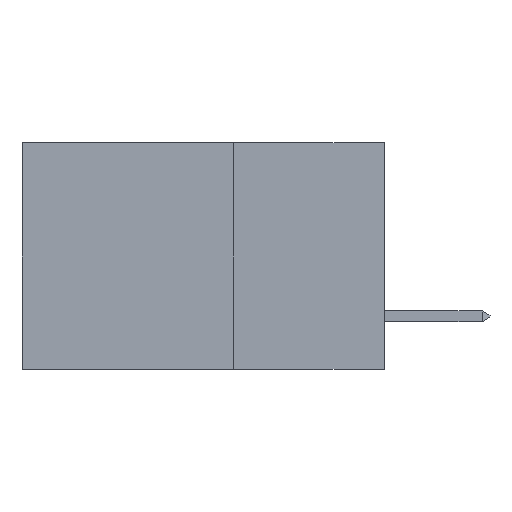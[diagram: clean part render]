
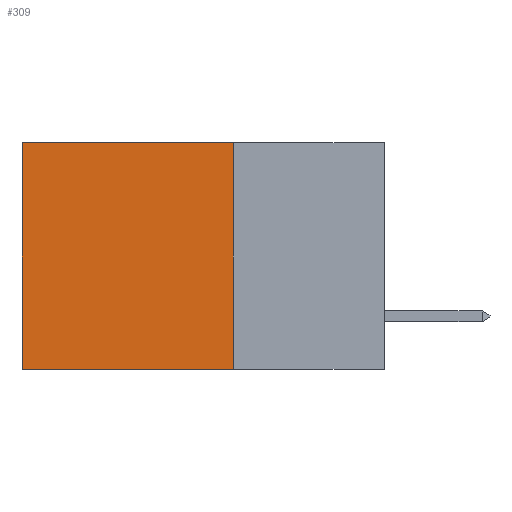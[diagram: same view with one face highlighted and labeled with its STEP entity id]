
A CAD part, left-side view. The second image highlights one B-rep face of the part: STEP entity #309.
In plain terms, the highlighted planar face has unit normal (-1, 0, 0).
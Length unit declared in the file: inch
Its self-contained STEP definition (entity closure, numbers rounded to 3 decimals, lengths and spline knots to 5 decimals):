
#145 = EDGE_CURVE ( 'NONE', #9549, #3495, #621, .T. ) ;
#281 = ORIENTED_EDGE ( 'NONE', *, *, #145, .T. ) ;
#309 = ADVANCED_FACE ( 'NONE', ( #3545 ), #6428, .F. ) ;
#405 = DIRECTION ( 'NONE',  ( 1., 0., 0. ) ) ;
#621 = LINE ( 'NONE', #3149, #6373 ) ;
#1084 = DIRECTION ( 'NONE',  ( 0., 0., -1. ) ) ;
#1146 = ORIENTED_EDGE ( 'NONE', *, *, #4583, .T. ) ;
#1243 = VECTOR ( 'NONE', #5095, 39.37008 ) ;
#1458 = LINE ( 'NONE', #4060, #7192 ) ;
#1569 = LINE ( 'NONE', #3589, #6022 ) ;
#2147 = ORIENTED_EDGE ( 'NONE', *, *, #7926, .F. ) ;
#2743 = DIRECTION ( 'NONE',  ( 0., 0., -1. ) ) ;
#2955 = DIRECTION ( 'NONE',  ( 0., 0., -1. ) ) ;
#3149 = CARTESIAN_POINT ( 'NONE',  ( 0.2875, 0.6, -0.375 ) ) ;
#3495 = VERTEX_POINT ( 'NONE', #4657 ) ;
#3545 = FACE_OUTER_BOUND ( 'NONE', #7083, .T. ) ;
#3589 = CARTESIAN_POINT ( 'NONE',  ( 0.2875, 0.25, -0.375 ) ) ;
#4060 = CARTESIAN_POINT ( 'NONE',  ( 0.2875, 0.25, -0.375 ) ) ;
#4084 = CARTESIAN_POINT ( 'NONE',  ( 0.2875, 0.6, 0. ) ) ;
#4092 = CARTESIAN_POINT ( 'NONE',  ( 0.2875, 0.25, 0. ) ) ;
#4281 = VERTEX_POINT ( 'NONE', #8550 ) ;
#4338 = CARTESIAN_POINT ( 'NONE',  ( 0.2875, 0.25, 0. ) ) ;
#4583 = EDGE_CURVE ( 'NONE', #8973, #9549, #5475, .T. ) ;
#4657 = CARTESIAN_POINT ( 'NONE',  ( 0.2875, 0.6, -0.375 ) ) ;
#4826 = DIRECTION ( 'NONE',  ( 0., 1., 0. ) ) ;
#4952 = CARTESIAN_POINT ( 'NONE',  ( 0.2875, 0.25, -0.375 ) ) ;
#5095 = DIRECTION ( 'NONE',  ( 0., 1., 0. ) ) ;
#5475 = LINE ( 'NONE', #4338, #1243 ) ;
#5564 = AXIS2_PLACEMENT_3D ( 'NONE', #4952, #405, #2743 ) ;
#6022 = VECTOR ( 'NONE', #2955, 39.37008 ) ;
#6373 = VECTOR ( 'NONE', #1084, 39.37008 ) ;
#6428 = PLANE ( 'NONE',  #5564 ) ;
#6469 = EDGE_CURVE ( 'NONE', #8973, #4281, #1569, .T. ) ;
#7082 = ORIENTED_EDGE ( 'NONE', *, *, #6469, .F. ) ;
#7083 = EDGE_LOOP ( 'NONE', ( #281, #2147, #7082, #1146 ) ) ;
#7192 = VECTOR ( 'NONE', #4826, 39.37008 ) ;
#7926 = EDGE_CURVE ( 'NONE', #4281, #3495, #1458, .T. ) ;
#8550 = CARTESIAN_POINT ( 'NONE',  ( 0.2875, 0.25, -0.375 ) ) ;
#8973 = VERTEX_POINT ( 'NONE', #4092 ) ;
#9549 = VERTEX_POINT ( 'NONE', #4084 ) ;
